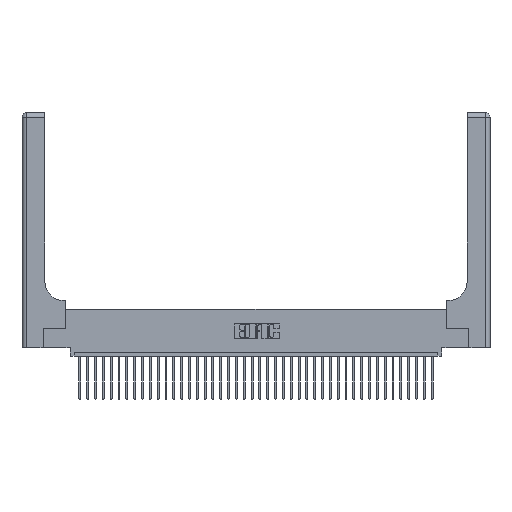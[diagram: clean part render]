
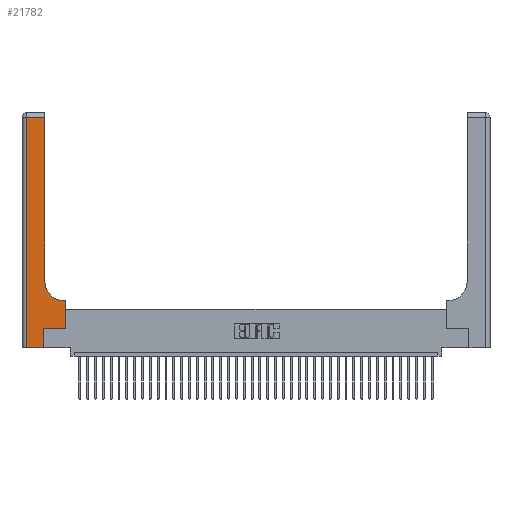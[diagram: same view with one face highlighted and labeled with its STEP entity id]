
A CAD part, top view. The second image highlights one B-rep face of the part: STEP entity #21782.
In plain terms, the highlighted planar face has unit normal (0, 0, 1).
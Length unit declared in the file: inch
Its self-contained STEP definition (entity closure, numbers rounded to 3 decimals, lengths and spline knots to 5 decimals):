
#266 = VERTEX_POINT ( 'NONE', #18701 ) ;
#347 = ORIENTED_EDGE ( 'NONE', *, *, #28746, .T. ) ;
#601 = DIRECTION ( 'NONE',  ( 0., -1., 0. ) ) ;
#1021 = LINE ( 'NONE', #17119, #27329 ) ;
#1096 = CARTESIAN_POINT ( 'NONE',  ( 0.06, 2.94, 0.37 ) ) ;
#1657 = DIRECTION ( 'NONE',  ( 0., 1., 0. ) ) ;
#1926 = AXIS2_PLACEMENT_3D ( 'NONE', #31559, #20831, #10176 ) ;
#2374 = VECTOR ( 'NONE', #23071, 39.37008 ) ;
#2443 = VECTOR ( 'NONE', #22411, 39.37008 ) ;
#2487 = ORIENTED_EDGE ( 'NONE', *, *, #36662, .T. ) ;
#3375 = EDGE_CURVE ( 'NONE', #14912, #8801, #1021, .T. ) ;
#3534 = ORIENTED_EDGE ( 'NONE', *, *, #21336, .T. ) ;
#3744 = CARTESIAN_POINT ( 'NONE',  ( 0.5415, 0.85, 0.37 ) ) ;
#4678 = CARTESIAN_POINT ( 'NONE',  ( 0.269, 0., 0.37 ) ) ;
#5283 = VECTOR ( 'NONE', #11432, 39.37008 ) ;
#5546 = EDGE_CURVE ( 'NONE', #266, #19402, #10533, .T. ) ;
#6058 = VERTEX_POINT ( 'NONE', #10326 ) ;
#6336 = VECTOR ( 'NONE', #7475, 39.37008 ) ;
#6469 = LINE ( 'NONE', #4678, #22665 ) ;
#6545 = VECTOR ( 'NONE', #601, 39.37008 ) ;
#6649 = AXIS2_PLACEMENT_3D ( 'NONE', #3744, #13480, #34814 ) ;
#7475 = DIRECTION ( 'NONE',  ( -1., 0., 0. ) ) ;
#8201 = CARTESIAN_POINT ( 'NONE',  ( 0.5415, 0.6, 0.37 ) ) ;
#8680 = ORIENTED_EDGE ( 'NONE', *, *, #36701, .T. ) ;
#8801 = VERTEX_POINT ( 'NONE', #16407 ) ;
#8996 = CARTESIAN_POINT ( 'NONE',  ( 0.5585, 0.25, 0.37 ) ) ;
#10176 = DIRECTION ( 'NONE',  ( -1., 0., 0. ) ) ;
#10326 = CARTESIAN_POINT ( 'NONE',  ( 0.06, 0., 0.37 ) ) ;
#10533 = LINE ( 'NONE', #35060, #2374 ) ;
#11432 = DIRECTION ( 'NONE',  ( 1., 0., 0. ) ) ;
#13302 = DIRECTION ( 'NONE',  ( 0., 1., 0. ) ) ;
#13480 = DIRECTION ( 'NONE',  ( 0., 0., -1. ) ) ;
#14068 = VERTEX_POINT ( 'NONE', #8996 ) ;
#14657 = LINE ( 'NONE', #31567, #6545 ) ;
#14912 = VERTEX_POINT ( 'NONE', #35406 ) ;
#15990 = ORIENTED_EDGE ( 'NONE', *, *, #3375, .T. ) ;
#16407 = CARTESIAN_POINT ( 'NONE',  ( 0.2915, 2.94, 0.37 ) ) ;
#16520 = ORIENTED_EDGE ( 'NONE', *, *, #31139, .T. ) ;
#16682 = ORIENTED_EDGE ( 'NONE', *, *, #32296, .T. ) ;
#16999 = EDGE_CURVE ( 'NONE', #35664, #14068, #35299, .T. ) ;
#17119 = CARTESIAN_POINT ( 'NONE',  ( 0.2915, 3., 0.37 ) ) ;
#18531 = VERTEX_POINT ( 'NONE', #28949 ) ;
#18611 = LINE ( 'NONE', #37437, #2443 ) ;
#18701 = CARTESIAN_POINT ( 'NONE',  ( 0.5585, 0.6, 0.37 ) ) ;
#19402 = VERTEX_POINT ( 'NONE', #8201 ) ;
#20136 = VERTEX_POINT ( 'NONE', #1096 ) ;
#20182 = CARTESIAN_POINT ( 'NONE',  ( 0.269, 0.25, 0.37 ) ) ;
#20831 = DIRECTION ( 'NONE',  ( 0., 0., -1. ) ) ;
#21336 = EDGE_CURVE ( 'NONE', #20136, #6058, #14657, .T. ) ;
#21782 = ADVANCED_FACE ( 'NONE', ( #26080 ), #37496, .F. ) ;
#22411 = DIRECTION ( 'NONE',  ( 0., 1., 0. ) ) ;
#22665 = VECTOR ( 'NONE', #13302, 39.37008 ) ;
#23071 = DIRECTION ( 'NONE',  ( -1., 0., 0. ) ) ;
#23586 = DIRECTION ( 'NONE',  ( 1., 0., 0. ) ) ;
#25892 = ORIENTED_EDGE ( 'NONE', *, *, #5546, .T. ) ;
#26080 = FACE_OUTER_BOUND ( 'NONE', #26335, .T. ) ;
#26335 = EDGE_LOOP ( 'NONE', ( #15990, #16520, #3534, #8680, #2487, #28647, #16682, #25892, #347 ) ) ;
#26548 = VECTOR ( 'NONE', #23586, 39.37008 ) ;
#26760 = CARTESIAN_POINT ( 'NONE',  ( 0.269, 0.25, 0.37 ) ) ;
#27329 = VECTOR ( 'NONE', #1657, 39.37008 ) ;
#28420 = LINE ( 'NONE', #38458, #26548 ) ;
#28647 = ORIENTED_EDGE ( 'NONE', *, *, #16999, .T. ) ;
#28746 = EDGE_CURVE ( 'NONE', #19402, #14912, #39150, .T. ) ;
#28920 = CARTESIAN_POINT ( 'NONE',  ( 0., 2.94, 0.37 ) ) ;
#28949 = CARTESIAN_POINT ( 'NONE',  ( 0.269, 0., 0.37 ) ) ;
#31139 = EDGE_CURVE ( 'NONE', #8801, #20136, #36790, .T. ) ;
#31559 = CARTESIAN_POINT ( 'NONE',  ( 0., 3., 0.37 ) ) ;
#31567 = CARTESIAN_POINT ( 'NONE',  ( 0.06, 3., 0.37 ) ) ;
#32296 = EDGE_CURVE ( 'NONE', #14068, #266, #18611, .T. ) ;
#34814 = DIRECTION ( 'NONE',  ( 1., 0., 0. ) ) ;
#35060 = CARTESIAN_POINT ( 'NONE',  ( 0.2915, 0.6, 0.37 ) ) ;
#35299 = LINE ( 'NONE', #20182, #5283 ) ;
#35406 = CARTESIAN_POINT ( 'NONE',  ( 0.2915, 0.85, 0.37 ) ) ;
#35664 = VERTEX_POINT ( 'NONE', #26760 ) ;
#36662 = EDGE_CURVE ( 'NONE', #18531, #35664, #6469, .T. ) ;
#36701 = EDGE_CURVE ( 'NONE', #6058, #18531, #28420, .T. ) ;
#36790 = LINE ( 'NONE', #28920, #6336 ) ;
#37437 = CARTESIAN_POINT ( 'NONE',  ( 0.5585, 0.25, 0.37 ) ) ;
#37496 = PLANE ( 'NONE',  #1926 ) ;
#38458 = CARTESIAN_POINT ( 'NONE',  ( 0., 0., 0.37 ) ) ;
#39150 = CIRCLE ( 'NONE', #6649, 0.25 ) ;
